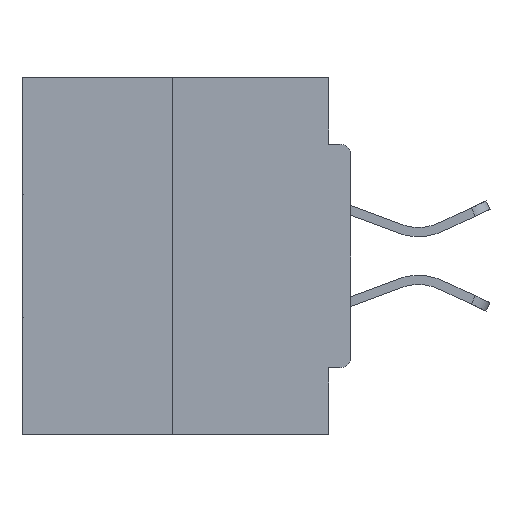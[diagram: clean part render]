
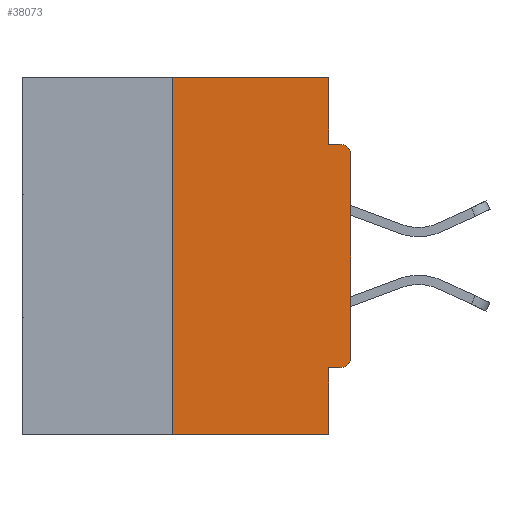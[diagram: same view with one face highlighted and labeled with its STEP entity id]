
A CAD part, left-side view. The second image highlights one B-rep face of the part: STEP entity #38073.
In plain terms, the highlighted planar face has unit normal (-1, 0, 0).
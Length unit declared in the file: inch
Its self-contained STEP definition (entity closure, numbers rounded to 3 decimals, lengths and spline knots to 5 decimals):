
#142 = CARTESIAN_POINT ( 'NONE',  ( 0., 0.031, 0. ) ) ;
#292 = CARTESIAN_POINT ( 'NONE',  ( 0., 0.015, -0.0935 ) ) ;
#903 = VERTEX_POINT ( 'NONE', #5038 ) ;
#913 = ORIENTED_EDGE ( 'NONE', *, *, #4727, .F. ) ;
#2692 = DIRECTION ( 'NONE',  ( 0., 0., -1. ) ) ;
#2794 = LINE ( 'NONE', #16150, #20445 ) ;
#3643 = CARTESIAN_POINT ( 'NONE',  ( 0., 0.46, -0.5 ) ) ;
#3656 = DIRECTION ( 'NONE',  ( 0., -1., 0. ) ) ;
#4058 = EDGE_CURVE ( 'NONE', #21427, #5070, #26057, .T. ) ;
#4159 = LINE ( 'NONE', #13529, #4657 ) ;
#4370 = CARTESIAN_POINT ( 'NONE',  ( 0., 0.25, 0. ) ) ;
#4429 = AXIS2_PLACEMENT_3D ( 'NONE', #30398, #18724, #18855 ) ;
#4657 = VECTOR ( 'NONE', #34247, 39.37008 ) ;
#4727 = EDGE_CURVE ( 'NONE', #5232, #34256, #19958, .T. ) ;
#4842 = CIRCLE ( 'NONE', #24114, 0.015 ) ;
#4851 = ORIENTED_EDGE ( 'NONE', *, *, #4058, .F. ) ;
#5038 = CARTESIAN_POINT ( 'NONE',  ( 0., 0., -0.1085 ) ) ;
#5070 = VERTEX_POINT ( 'NONE', #20356 ) ;
#5232 = VERTEX_POINT ( 'NONE', #12076 ) ;
#5816 = VERTEX_POINT ( 'NONE', #26710 ) ;
#6122 = LINE ( 'NONE', #31125, #25587 ) ;
#6896 = EDGE_LOOP ( 'NONE', ( #913, #12190, #22860, #4851, #29218, #27153, #29881, #13806, #17591, #25037 ) ) ;
#7642 = CARTESIAN_POINT ( 'NONE',  ( 0., 0., -0.3915 ) ) ;
#9658 = PLANE ( 'NONE',  #4429 ) ;
#9964 = EDGE_CURVE ( 'NONE', #5816, #5232, #29390, .T. ) ;
#10279 = AXIS2_PLACEMENT_3D ( 'NONE', #29472, #11985, #14971 ) ;
#11373 = VECTOR ( 'NONE', #2692, 39.37008 ) ;
#11668 = EDGE_CURVE ( 'NONE', #18022, #903, #6122, .T. ) ;
#11985 = DIRECTION ( 'NONE',  ( -1., 0., 0. ) ) ;
#12076 = CARTESIAN_POINT ( 'NONE',  ( 0., 0.25, 0. ) ) ;
#12190 = ORIENTED_EDGE ( 'NONE', *, *, #9964, .F. ) ;
#13360 = VERTEX_POINT ( 'NONE', #18937 ) ;
#13529 = CARTESIAN_POINT ( 'NONE',  ( 0., 0., -0.0935 ) ) ;
#13806 = ORIENTED_EDGE ( 'NONE', *, *, #29121, .T. ) ;
#14634 = LINE ( 'NONE', #142, #11373 ) ;
#14971 = DIRECTION ( 'NONE',  ( 0., 0., -1. ) ) ;
#16150 = CARTESIAN_POINT ( 'NONE',  ( 0., 0., -0.4065 ) ) ;
#16256 = CARTESIAN_POINT ( 'NONE',  ( 0., 0.031, -0.5 ) ) ;
#16650 = CARTESIAN_POINT ( 'NONE',  ( 0., 0.031, 0. ) ) ;
#17591 = ORIENTED_EDGE ( 'NONE', *, *, #27668, .F. ) ;
#18022 = VERTEX_POINT ( 'NONE', #7642 ) ;
#18597 = DIRECTION ( 'NONE',  ( 0., -1., 0. ) ) ;
#18724 = DIRECTION ( 'NONE',  ( 1., 0., 0. ) ) ;
#18809 = LINE ( 'NONE', #3643, #27141 ) ;
#18829 = EDGE_CURVE ( 'NONE', #13360, #21427, #2794, .T. ) ;
#18855 = DIRECTION ( 'NONE',  ( 0., 0., -1. ) ) ;
#18937 = CARTESIAN_POINT ( 'NONE',  ( 0., 0.015, -0.4065 ) ) ;
#19285 = CIRCLE ( 'NONE', #10279, 0.015 ) ;
#19958 = LINE ( 'NONE', #27300, #24600 ) ;
#20020 = VERTEX_POINT ( 'NONE', #292 ) ;
#20356 = CARTESIAN_POINT ( 'NONE',  ( 0., 0.031, -0.5 ) ) ;
#20445 = VECTOR ( 'NONE', #24661, 39.37008 ) ;
#20762 = DIRECTION ( 'NONE',  ( -1., 0., 0. ) ) ;
#21427 = VERTEX_POINT ( 'NONE', #26747 ) ;
#21949 = EDGE_CURVE ( 'NONE', #34256, #34040, #14634, .T. ) ;
#22860 = ORIENTED_EDGE ( 'NONE', *, *, #38082, .T. ) ;
#23943 = EDGE_CURVE ( 'NONE', #13360, #18022, #19285, .T. ) ;
#24114 = AXIS2_PLACEMENT_3D ( 'NONE', #26718, #20762, #29714 ) ;
#24600 = VECTOR ( 'NONE', #3656, 39.37008 ) ;
#24661 = DIRECTION ( 'NONE',  ( 0., 1., 0. ) ) ;
#25037 = ORIENTED_EDGE ( 'NONE', *, *, #21949, .F. ) ;
#25122 = VECTOR ( 'NONE', #37058, 39.37008 ) ;
#25587 = VECTOR ( 'NONE', #36545, 39.37008 ) ;
#25744 = FACE_OUTER_BOUND ( 'NONE', #6896, .T. ) ;
#26057 = LINE ( 'NONE', #16256, #25122 ) ;
#26613 = CARTESIAN_POINT ( 'NONE',  ( 0., 0.031, -0.0935 ) ) ;
#26710 = CARTESIAN_POINT ( 'NONE',  ( 0., 0.25, -0.5 ) ) ;
#26718 = CARTESIAN_POINT ( 'NONE',  ( 0., 0.015, -0.1085 ) ) ;
#26747 = CARTESIAN_POINT ( 'NONE',  ( 0., 0.031, -0.4065 ) ) ;
#27141 = VECTOR ( 'NONE', #18597, 39.37008 ) ;
#27153 = ORIENTED_EDGE ( 'NONE', *, *, #23943, .T. ) ;
#27300 = CARTESIAN_POINT ( 'NONE',  ( 0., 0.46, 0. ) ) ;
#27668 = EDGE_CURVE ( 'NONE', #34040, #20020, #4159, .T. ) ;
#28130 = DIRECTION ( 'NONE',  ( 0., 0., 1. ) ) ;
#29121 = EDGE_CURVE ( 'NONE', #903, #20020, #4842, .T. ) ;
#29218 = ORIENTED_EDGE ( 'NONE', *, *, #18829, .F. ) ;
#29390 = LINE ( 'NONE', #4370, #34949 ) ;
#29472 = CARTESIAN_POINT ( 'NONE',  ( 0., 0.015, -0.3915 ) ) ;
#29714 = DIRECTION ( 'NONE',  ( 0., 0., -1. ) ) ;
#29881 = ORIENTED_EDGE ( 'NONE', *, *, #11668, .T. ) ;
#30398 = CARTESIAN_POINT ( 'NONE',  ( 0., 0.46, 0. ) ) ;
#31125 = CARTESIAN_POINT ( 'NONE',  ( 0., 0., 0. ) ) ;
#34040 = VERTEX_POINT ( 'NONE', #26613 ) ;
#34247 = DIRECTION ( 'NONE',  ( 0., -1., 0. ) ) ;
#34256 = VERTEX_POINT ( 'NONE', #16650 ) ;
#34949 = VECTOR ( 'NONE', #28130, 39.37008 ) ;
#36545 = DIRECTION ( 'NONE',  ( 0., 0., 1. ) ) ;
#37058 = DIRECTION ( 'NONE',  ( 0., 0., -1. ) ) ;
#38073 = ADVANCED_FACE ( 'NONE', ( #25744 ), #9658, .F. ) ;
#38082 = EDGE_CURVE ( 'NONE', #5816, #5070, #18809, .T. ) ;
